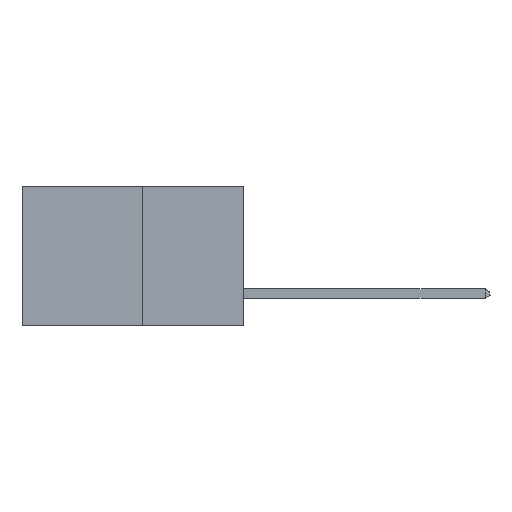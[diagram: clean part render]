
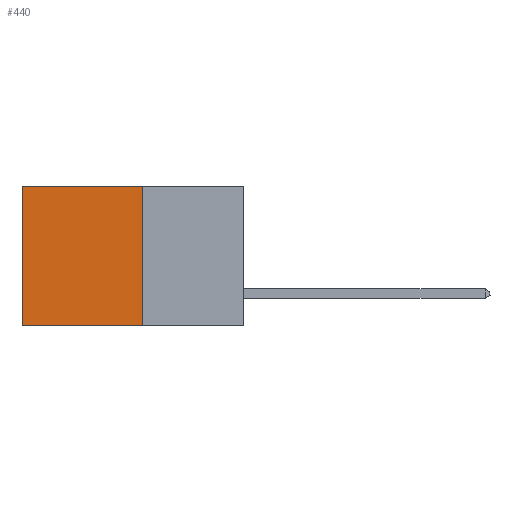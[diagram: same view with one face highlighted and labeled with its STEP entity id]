
A CAD part, left-side view. The second image highlights one B-rep face of the part: STEP entity #440.
In plain terms, the highlighted planar face has unit normal (-1, 0, 0).
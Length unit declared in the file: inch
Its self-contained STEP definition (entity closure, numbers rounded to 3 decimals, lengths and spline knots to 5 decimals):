
#37 = VERTEX_POINT ( 'NONE', #10791 ) ;
#336 = ORIENTED_EDGE ( 'NONE', *, *, #8115, .F. ) ;
#430 = CARTESIAN_POINT ( 'NONE',  ( 0.277, 0.59, -0.37 ) ) ;
#440 = ADVANCED_FACE ( 'NONE', ( #2656 ), #8251, .F. ) ;
#1501 = VECTOR ( 'NONE', #13446, 39.37008 ) ;
#1926 = CARTESIAN_POINT ( 'NONE',  ( 0.277, 0.59, -0.37 ) ) ;
#2606 = VECTOR ( 'NONE', #4118, 39.37008 ) ;
#2656 = FACE_OUTER_BOUND ( 'NONE', #3433, .T. ) ;
#2667 = LINE ( 'NONE', #430, #11620 ) ;
#2915 = ORIENTED_EDGE ( 'NONE', *, *, #8093, .T. ) ;
#3433 = EDGE_LOOP ( 'NONE', ( #4222, #336, #12539, #2915 ) ) ;
#4118 = DIRECTION ( 'NONE',  ( 0., 1., 0. ) ) ;
#4158 = CARTESIAN_POINT ( 'NONE',  ( 0.277, 0.27, 0. ) ) ;
#4222 = ORIENTED_EDGE ( 'NONE', *, *, #12065, .T. ) ;
#4298 = DIRECTION ( 'NONE',  ( 0., 0., -1. ) ) ;
#4430 = LINE ( 'NONE', #5105, #13611 ) ;
#5043 = LINE ( 'NONE', #4158, #2606 ) ;
#5105 = CARTESIAN_POINT ( 'NONE',  ( 0.277, 0.27, -0.37 ) ) ;
#5727 = AXIS2_PLACEMENT_3D ( 'NONE', #9160, #9671, #9283 ) ;
#6108 = VERTEX_POINT ( 'NONE', #9888 ) ;
#6372 = DIRECTION ( 'NONE',  ( 0., 0., -1. ) ) ;
#7560 = VERTEX_POINT ( 'NONE', #1926 ) ;
#8093 = EDGE_CURVE ( 'NONE', #6108, #14471, #5043, .T. ) ;
#8115 = EDGE_CURVE ( 'NONE', #37, #7560, #13809, .T. ) ;
#8251 = PLANE ( 'NONE',  #5727 ) ;
#8749 = EDGE_CURVE ( 'NONE', #6108, #37, #4430, .T. ) ;
#9160 = CARTESIAN_POINT ( 'NONE',  ( 0.277, 0.27, -0.37 ) ) ;
#9283 = DIRECTION ( 'NONE',  ( 0., 0., -1. ) ) ;
#9671 = DIRECTION ( 'NONE',  ( 1., 0., 0. ) ) ;
#9888 = CARTESIAN_POINT ( 'NONE',  ( 0.277, 0.27, 0. ) ) ;
#10791 = CARTESIAN_POINT ( 'NONE',  ( 0.277, 0.27, -0.37 ) ) ;
#10884 = CARTESIAN_POINT ( 'NONE',  ( 0.277, 0.59, 0. ) ) ;
#11620 = VECTOR ( 'NONE', #6372, 39.37008 ) ;
#12065 = EDGE_CURVE ( 'NONE', #14471, #7560, #2667, .T. ) ;
#12539 = ORIENTED_EDGE ( 'NONE', *, *, #8749, .F. ) ;
#13446 = DIRECTION ( 'NONE',  ( 0., 1., 0. ) ) ;
#13611 = VECTOR ( 'NONE', #4298, 39.37008 ) ;
#13651 = CARTESIAN_POINT ( 'NONE',  ( 0.277, 0.27, -0.37 ) ) ;
#13809 = LINE ( 'NONE', #13651, #1501 ) ;
#14471 = VERTEX_POINT ( 'NONE', #10884 ) ;
